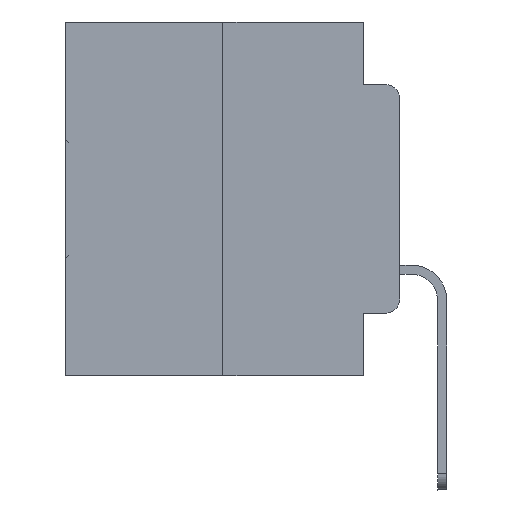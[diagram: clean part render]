
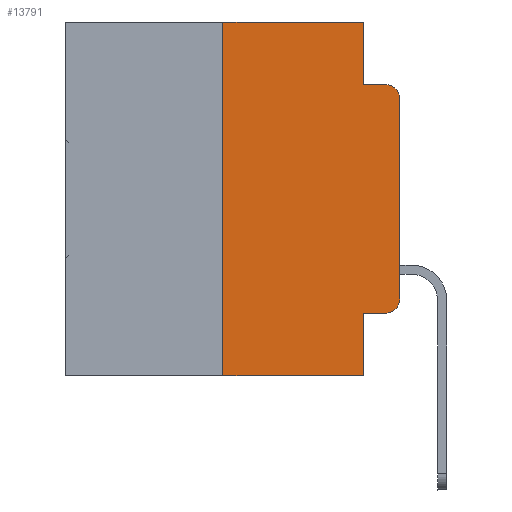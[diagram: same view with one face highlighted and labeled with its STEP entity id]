
A CAD part, left-side view. The second image highlights one B-rep face of the part: STEP entity #13791.
In plain terms, the highlighted planar face has unit normal (-1, 0, 0).
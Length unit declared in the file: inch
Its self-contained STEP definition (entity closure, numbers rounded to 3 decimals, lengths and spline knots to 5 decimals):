
#35 = VECTOR ( 'NONE', #20383, 39.37008 ) ;
#90 = DIRECTION ( 'NONE',  ( -1., 0., 0. ) ) ;
#682 = ORIENTED_EDGE ( 'NONE', *, *, #8360, .F. ) ;
#837 = ORIENTED_EDGE ( 'NONE', *, *, #2298, .F. ) ;
#915 = VERTEX_POINT ( 'NONE', #10694 ) ;
#966 = VERTEX_POINT ( 'NONE', #25073 ) ;
#1487 = AXIS2_PLACEMENT_3D ( 'NONE', #14999, #90, #17198 ) ;
#1674 = EDGE_CURVE ( 'NONE', #21247, #915, #15023, .T. ) ;
#2298 = EDGE_CURVE ( 'NONE', #2980, #19599, #12767, .T. ) ;
#2605 = CARTESIAN_POINT ( 'NONE',  ( 0., 0.473, -0.5 ) ) ;
#2980 = VERTEX_POINT ( 'NONE', #26268 ) ;
#2993 = EDGE_CURVE ( 'NONE', #21534, #13967, #12043, .T. ) ;
#3052 = CARTESIAN_POINT ( 'NONE',  ( 0., 0.051, 0. ) ) ;
#3211 = VECTOR ( 'NONE', #13115, 39.37008 ) ;
#3605 = DIRECTION ( 'NONE',  ( 0., 0., -1. ) ) ;
#5102 = CARTESIAN_POINT ( 'NONE',  ( 0., 0.051, 0. ) ) ;
#5106 = DIRECTION ( 'NONE',  ( 0., 0., -1. ) ) ;
#5665 = CARTESIAN_POINT ( 'NONE',  ( 0., 0.02, -0.1085 ) ) ;
#6085 = LINE ( 'NONE', #8594, #20758 ) ;
#6273 = LINE ( 'NONE', #10835, #35 ) ;
#6470 = EDGE_CURVE ( 'NONE', #915, #26838, #6085, .T. ) ;
#6622 = DIRECTION ( 'NONE',  ( 1., 0., 0. ) ) ;
#6682 = CARTESIAN_POINT ( 'NONE',  ( 0., 0.473, 0. ) ) ;
#6839 = CARTESIAN_POINT ( 'NONE',  ( 0., 0., -0.1085 ) ) ;
#7300 = EDGE_LOOP ( 'NONE', ( #10674, #16319, #837, #25570, #22051, #682, #27278, #27150, #22107, #11421 ) ) ;
#7441 = DIRECTION ( 'NONE',  ( 0., 0., 1. ) ) ;
#7764 = DIRECTION ( 'NONE',  ( 0., -1., 0. ) ) ;
#7774 = DIRECTION ( 'NONE',  ( 0., 0., -1. ) ) ;
#7778 = LINE ( 'NONE', #3052, #21116 ) ;
#8360 = EDGE_CURVE ( 'NONE', #21534, #966, #24487, .T. ) ;
#8381 = CARTESIAN_POINT ( 'NONE',  ( 0., 0.051, -0.0885 ) ) ;
#8594 = CARTESIAN_POINT ( 'NONE',  ( 0., 0., 0. ) ) ;
#9809 = LINE ( 'NONE', #5102, #13441 ) ;
#10457 = VECTOR ( 'NONE', #21541, 39.37008 ) ;
#10674 = ORIENTED_EDGE ( 'NONE', *, *, #6470, .T. ) ;
#10694 = CARTESIAN_POINT ( 'NONE',  ( 0., 0., -0.3915 ) ) ;
#10835 = CARTESIAN_POINT ( 'NONE',  ( 0., 0.051, -0.4115 ) ) ;
#10868 = DIRECTION ( 'NONE',  ( 0., 0., -1. ) ) ;
#11276 = VECTOR ( 'NONE', #7441, 39.37008 ) ;
#11327 = CARTESIAN_POINT ( 'NONE',  ( 0., 0.02, -0.4115 ) ) ;
#11421 = ORIENTED_EDGE ( 'NONE', *, *, #1674, .T. ) ;
#11994 = CARTESIAN_POINT ( 'NONE',  ( 0., 0.25, 0. ) ) ;
#12043 = LINE ( 'NONE', #2605, #3211 ) ;
#12353 = VERTEX_POINT ( 'NONE', #21636 ) ;
#12767 = LINE ( 'NONE', #8381, #17942 ) ;
#13115 = DIRECTION ( 'NONE',  ( 0., -1., 0. ) ) ;
#13441 = VECTOR ( 'NONE', #7774, 39.37008 ) ;
#13675 = CARTESIAN_POINT ( 'NONE',  ( 0., 0.473, 0. ) ) ;
#13791 = ADVANCED_FACE ( 'NONE', ( #18683 ), #20871, .F. ) ;
#13967 = VERTEX_POINT ( 'NONE', #26178 ) ;
#14208 = CARTESIAN_POINT ( 'NONE',  ( 0., 0.051, 0. ) ) ;
#14242 = EDGE_CURVE ( 'NONE', #12353, #21247, #6273, .T. ) ;
#14999 = CARTESIAN_POINT ( 'NONE',  ( 0., 0.02, -0.3915 ) ) ;
#15023 = CIRCLE ( 'NONE', #1487, 0.02 ) ;
#16319 = ORIENTED_EDGE ( 'NONE', *, *, #30145, .T. ) ;
#17198 = DIRECTION ( 'NONE',  ( 0., 0., -1. ) ) ;
#17539 = DIRECTION ( 'NONE',  ( 0., 0., 1. ) ) ;
#17942 = VECTOR ( 'NONE', #7764, 39.37008 ) ;
#18159 = CIRCLE ( 'NONE', #28147, 0.02 ) ;
#18389 = CARTESIAN_POINT ( 'NONE',  ( 0., 0.02, -0.0885 ) ) ;
#18683 = FACE_OUTER_BOUND ( 'NONE', #7300, .T. ) ;
#19599 = VERTEX_POINT ( 'NONE', #18389 ) ;
#20342 = EDGE_CURVE ( 'NONE', #966, #30920, #30048, .T. ) ;
#20383 = DIRECTION ( 'NONE',  ( 0., -1., 0. ) ) ;
#20441 = EDGE_CURVE ( 'NONE', #30920, #2980, #9809, .T. ) ;
#20758 = VECTOR ( 'NONE', #17539, 39.37008 ) ;
#20871 = PLANE ( 'NONE',  #28040 ) ;
#21116 = VECTOR ( 'NONE', #5106, 39.37008 ) ;
#21247 = VERTEX_POINT ( 'NONE', #11327 ) ;
#21534 = VERTEX_POINT ( 'NONE', #26798 ) ;
#21541 = DIRECTION ( 'NONE',  ( 0., -1., 0. ) ) ;
#21636 = CARTESIAN_POINT ( 'NONE',  ( 0., 0.051, -0.4115 ) ) ;
#22051 = ORIENTED_EDGE ( 'NONE', *, *, #20342, .F. ) ;
#22105 = DIRECTION ( 'NONE',  ( -1., 0., 0. ) ) ;
#22107 = ORIENTED_EDGE ( 'NONE', *, *, #14242, .T. ) ;
#24487 = LINE ( 'NONE', #11994, #11276 ) ;
#25073 = CARTESIAN_POINT ( 'NONE',  ( 0., 0.25, 0. ) ) ;
#25570 = ORIENTED_EDGE ( 'NONE', *, *, #20441, .F. ) ;
#26178 = CARTESIAN_POINT ( 'NONE',  ( 0., 0.051, -0.5 ) ) ;
#26268 = CARTESIAN_POINT ( 'NONE',  ( 0., 0.051, -0.0885 ) ) ;
#26798 = CARTESIAN_POINT ( 'NONE',  ( 0., 0.25, -0.5 ) ) ;
#26838 = VERTEX_POINT ( 'NONE', #6839 ) ;
#27150 = ORIENTED_EDGE ( 'NONE', *, *, #28196, .F. ) ;
#27278 = ORIENTED_EDGE ( 'NONE', *, *, #2993, .T. ) ;
#28040 = AXIS2_PLACEMENT_3D ( 'NONE', #13675, #6622, #10868 ) ;
#28147 = AXIS2_PLACEMENT_3D ( 'NONE', #5665, #22105, #3605 ) ;
#28196 = EDGE_CURVE ( 'NONE', #12353, #13967, #7778, .T. ) ;
#30048 = LINE ( 'NONE', #6682, #10457 ) ;
#30145 = EDGE_CURVE ( 'NONE', #26838, #19599, #18159, .T. ) ;
#30920 = VERTEX_POINT ( 'NONE', #14208 ) ;
